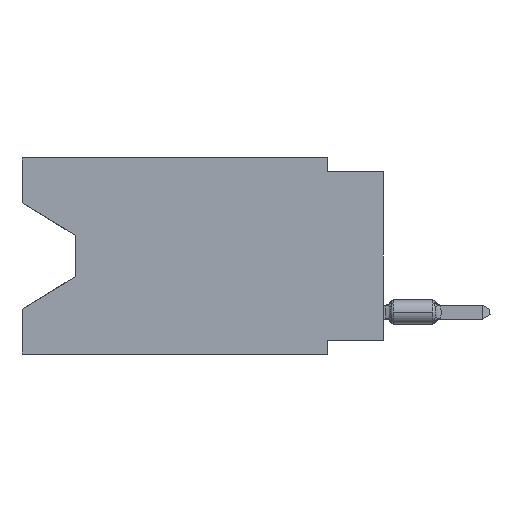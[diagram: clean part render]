
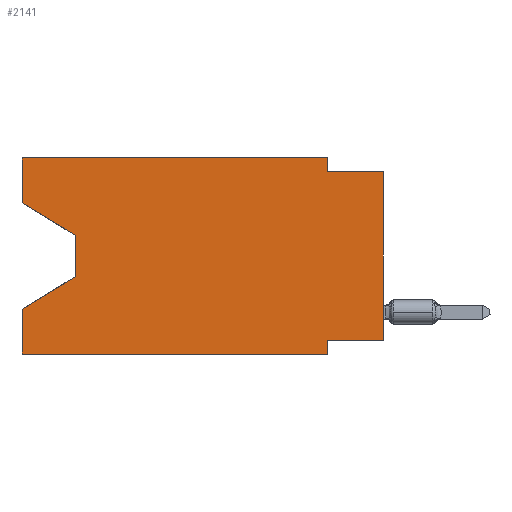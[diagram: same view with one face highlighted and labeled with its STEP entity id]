
A CAD part, left-side view. The second image highlights one B-rep face of the part: STEP entity #2141.
In plain terms, the highlighted planar face has unit normal (-1, 0, 0).
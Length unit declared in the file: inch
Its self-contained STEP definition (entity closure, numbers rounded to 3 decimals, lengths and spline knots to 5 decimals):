
#1081 = EDGE_CURVE ( 'NONE', #4571, #28978, #10235, .T. ) ;
#1521 = VECTOR ( 'NONE', #8137, 39.37008 ) ;
#1730 = DIRECTION ( 'NONE',  ( 0., -1., 0. ) ) ;
#2058 = LINE ( 'NONE', #11140, #16209 ) ;
#2141 = ADVANCED_FACE ( 'NONE', ( #28310 ), #8259, .F. ) ;
#2673 = VECTOR ( 'NONE', #13051, 39.37008 ) ;
#3054 = CARTESIAN_POINT ( 'NONE',  ( 0., 0.1, -0.325 ) ) ;
#3431 = DIRECTION ( 'NONE',  ( 0., 0., 1. ) ) ;
#3459 = LINE ( 'NONE', #31842, #34159 ) ;
#3614 = VERTEX_POINT ( 'NONE', #35620 ) ;
#4571 = VERTEX_POINT ( 'NONE', #34182 ) ;
#4779 = DIRECTION ( 'NONE',  ( 0., 0., -1. ) ) ;
#4869 = LINE ( 'NONE', #27147, #34101 ) ;
#4985 = DIRECTION ( 'NONE',  ( 0., 0., 1. ) ) ;
#5356 = VERTEX_POINT ( 'NONE', #12929 ) ;
#6848 = VERTEX_POINT ( 'NONE', #10561 ) ;
#7470 = DIRECTION ( 'NONE',  ( 0., 1., 0. ) ) ;
#7681 = LINE ( 'NONE', #18996, #10425 ) ;
#7768 = ORIENTED_EDGE ( 'NONE', *, *, #33747, .T. ) ;
#8137 = DIRECTION ( 'NONE',  ( 0., 0., -1. ) ) ;
#8259 = PLANE ( 'NONE',  #18051 ) ;
#8633 = LINE ( 'NONE', #20297, #34666 ) ;
#9625 = CARTESIAN_POINT ( 'NONE',  ( 0., 0.55, -0.138 ) ) ;
#10235 = LINE ( 'NONE', #10605, #18323 ) ;
#10425 = VECTOR ( 'NONE', #30325, 39.37008 ) ;
#10561 = CARTESIAN_POINT ( 'NONE',  ( 0., 0.645, 0. ) ) ;
#10605 = CARTESIAN_POINT ( 'NONE',  ( 0., 0., -0.325 ) ) ;
#10869 = VERTEX_POINT ( 'NONE', #9625 ) ;
#11140 = CARTESIAN_POINT ( 'NONE',  ( 0., 0.55, -0.212 ) ) ;
#11727 = VERTEX_POINT ( 'NONE', #13499 ) ;
#11898 = LINE ( 'NONE', #17665, #15642 ) ;
#12166 = ORIENTED_EDGE ( 'NONE', *, *, #29537, .F. ) ;
#12929 = CARTESIAN_POINT ( 'NONE',  ( 0., 0.1, -0.35 ) ) ;
#12940 = CARTESIAN_POINT ( 'NONE',  ( 0., 0.55, -0.138 ) ) ;
#13051 = DIRECTION ( 'NONE',  ( 0., -1., 0. ) ) ;
#13437 = CARTESIAN_POINT ( 'NONE',  ( 0., 0.645, -0.08025 ) ) ;
#13499 = CARTESIAN_POINT ( 'NONE',  ( 0., 0.645, -0.26975 ) ) ;
#13932 = ORIENTED_EDGE ( 'NONE', *, *, #33559, .F. ) ;
#14554 = CARTESIAN_POINT ( 'NONE',  ( 0., 0.645, -0.08025 ) ) ;
#15642 = VECTOR ( 'NONE', #23223, 39.37008 ) ;
#15644 = ORIENTED_EDGE ( 'NONE', *, *, #34409, .F. ) ;
#16031 = EDGE_CURVE ( 'NONE', #21251, #11727, #2058, .T. ) ;
#16209 = VECTOR ( 'NONE', #24485, 39.37008 ) ;
#16308 = VECTOR ( 'NONE', #4779, 39.37008 ) ;
#17048 = LINE ( 'NONE', #33577, #1521 ) ;
#17053 = VERTEX_POINT ( 'NONE', #27009 ) ;
#17178 = DIRECTION ( 'NONE',  ( 0., -1., 0. ) ) ;
#17665 = CARTESIAN_POINT ( 'NONE',  ( 0., 0.1, 0. ) ) ;
#17674 = EDGE_CURVE ( 'NONE', #28270, #5356, #27168, .T. ) ;
#17766 = ORIENTED_EDGE ( 'NONE', *, *, #36409, .T. ) ;
#17903 = ORIENTED_EDGE ( 'NONE', *, *, #34945, .F. ) ;
#18051 = AXIS2_PLACEMENT_3D ( 'NONE', #21986, #36496, #25337 ) ;
#18323 = VECTOR ( 'NONE', #7470, 39.37008 ) ;
#18996 = CARTESIAN_POINT ( 'NONE',  ( 0., 0., 0. ) ) ;
#19338 = ORIENTED_EDGE ( 'NONE', *, *, #26461, .T. ) ;
#20086 = ORIENTED_EDGE ( 'NONE', *, *, #17674, .T. ) ;
#20297 = CARTESIAN_POINT ( 'NONE',  ( 0., 0.645, 0. ) ) ;
#20779 = VECTOR ( 'NONE', #4985, 39.37008 ) ;
#20906 = EDGE_LOOP ( 'NONE', ( #19338, #7768, #28599, #36584, #20086, #15644, #32736, #17766, #17903, #12166, #13932, #31224 ) ) ;
#21251 = VERTEX_POINT ( 'NONE', #36714 ) ;
#21594 = CARTESIAN_POINT ( 'NONE',  ( 0., 0.645, -0.35 ) ) ;
#21986 = CARTESIAN_POINT ( 'NONE',  ( 0., 0.645, 0. ) ) ;
#23223 = DIRECTION ( 'NONE',  ( 0., 0., -1. ) ) ;
#24258 = CARTESIAN_POINT ( 'NONE',  ( 0., 0.645, -0.35 ) ) ;
#24485 = DIRECTION ( 'NONE',  ( 0., 0.855, -0.519 ) ) ;
#25206 = LINE ( 'NONE', #33923, #20779 ) ;
#25324 = VERTEX_POINT ( 'NONE', #29954 ) ;
#25337 = DIRECTION ( 'NONE',  ( 0., 0., -1. ) ) ;
#26136 = EDGE_CURVE ( 'NONE', #28270, #11727, #25206, .T. ) ;
#26461 = EDGE_CURVE ( 'NONE', #27758, #10869, #32046, .T. ) ;
#27009 = CARTESIAN_POINT ( 'NONE',  ( 0., 0., -0.025 ) ) ;
#27147 = CARTESIAN_POINT ( 'NONE',  ( 0., 0.645, 0. ) ) ;
#27168 = LINE ( 'NONE', #21594, #2673 ) ;
#27407 = LINE ( 'NONE', #12940, #16308 ) ;
#27758 = VERTEX_POINT ( 'NONE', #14554 ) ;
#28270 = VERTEX_POINT ( 'NONE', #24258 ) ;
#28310 = FACE_OUTER_BOUND ( 'NONE', #20906, .T. ) ;
#28599 = ORIENTED_EDGE ( 'NONE', *, *, #16031, .T. ) ;
#28978 = VERTEX_POINT ( 'NONE', #3054 ) ;
#29537 = EDGE_CURVE ( 'NONE', #3614, #25324, #11898, .T. ) ;
#29954 = CARTESIAN_POINT ( 'NONE',  ( 0., 0.1, -0.025 ) ) ;
#30325 = DIRECTION ( 'NONE',  ( 0., 0., 1. ) ) ;
#31224 = ORIENTED_EDGE ( 'NONE', *, *, #33209, .F. ) ;
#31842 = CARTESIAN_POINT ( 'NONE',  ( 0., 0., -0.025 ) ) ;
#32046 = LINE ( 'NONE', #13437, #35021 ) ;
#32736 = ORIENTED_EDGE ( 'NONE', *, *, #1081, .F. ) ;
#33112 = DIRECTION ( 'NONE',  ( 0., -0.855, -0.519 ) ) ;
#33209 = EDGE_CURVE ( 'NONE', #27758, #6848, #8633, .T. ) ;
#33559 = EDGE_CURVE ( 'NONE', #6848, #3614, #4869, .T. ) ;
#33577 = CARTESIAN_POINT ( 'NONE',  ( 0., 0.1, -0.35 ) ) ;
#33747 = EDGE_CURVE ( 'NONE', #10869, #21251, #27407, .T. ) ;
#33923 = CARTESIAN_POINT ( 'NONE',  ( 0., 0.645, 0. ) ) ;
#34101 = VECTOR ( 'NONE', #1730, 39.37008 ) ;
#34159 = VECTOR ( 'NONE', #17178, 39.37008 ) ;
#34182 = CARTESIAN_POINT ( 'NONE',  ( 0., 0., -0.325 ) ) ;
#34409 = EDGE_CURVE ( 'NONE', #28978, #5356, #17048, .T. ) ;
#34666 = VECTOR ( 'NONE', #3431, 39.37008 ) ;
#34945 = EDGE_CURVE ( 'NONE', #25324, #17053, #3459, .T. ) ;
#35021 = VECTOR ( 'NONE', #33112, 39.37008 ) ;
#35620 = CARTESIAN_POINT ( 'NONE',  ( 0., 0.1, 0. ) ) ;
#36409 = EDGE_CURVE ( 'NONE', #4571, #17053, #7681, .T. ) ;
#36496 = DIRECTION ( 'NONE',  ( 1., 0., 0. ) ) ;
#36584 = ORIENTED_EDGE ( 'NONE', *, *, #26136, .F. ) ;
#36714 = CARTESIAN_POINT ( 'NONE',  ( 0., 0.55, -0.212 ) ) ;
